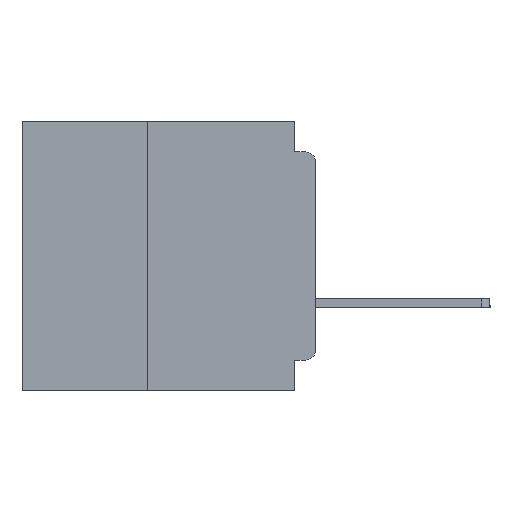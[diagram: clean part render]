
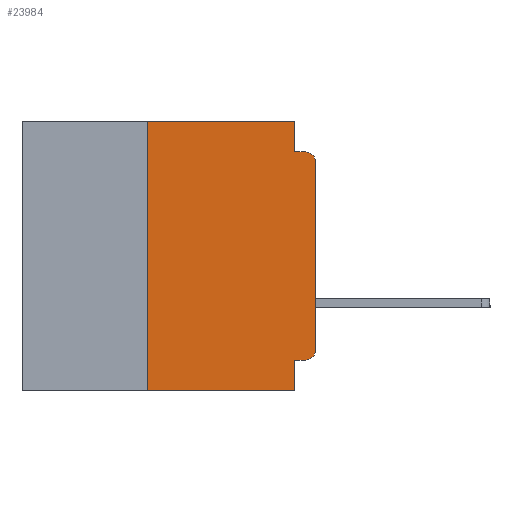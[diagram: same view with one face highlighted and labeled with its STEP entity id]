
A CAD part, left-side view. The second image highlights one B-rep face of the part: STEP entity #23984.
In plain terms, the highlighted planar face has unit normal (-1, 0, 0).
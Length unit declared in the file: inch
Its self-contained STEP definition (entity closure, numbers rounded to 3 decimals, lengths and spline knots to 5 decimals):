
#201 = ORIENTED_EDGE ( 'NONE', *, *, #36468, .T. ) ;
#619 = DIRECTION ( 'NONE',  ( 0., 1., 0. ) ) ;
#934 = CARTESIAN_POINT ( 'NONE',  ( 0., 0.25, 0. ) ) ;
#1139 = CARTESIAN_POINT ( 'NONE',  ( 0., 0.015, -0.355 ) ) ;
#1178 = CARTESIAN_POINT ( 'NONE',  ( 0., 0., -0.34 ) ) ;
#1828 = VERTEX_POINT ( 'NONE', #10863 ) ;
#1840 = CIRCLE ( 'NONE', #8574, 0.015 ) ;
#2480 = EDGE_CURVE ( 'NONE', #13129, #38058, #24101, .T. ) ;
#3026 = LINE ( 'NONE', #18519, #29274 ) ;
#3464 = LINE ( 'NONE', #41823, #29696 ) ;
#3977 = DIRECTION ( 'NONE',  ( 0., -1., 0. ) ) ;
#4245 = VERTEX_POINT ( 'NONE', #34113 ) ;
#4322 = CIRCLE ( 'NONE', #29673, 0.015 ) ;
#4446 = CARTESIAN_POINT ( 'NONE',  ( 0., 0.25, -0.4 ) ) ;
#4494 = DIRECTION ( 'NONE',  ( -1., 0., 0. ) ) ;
#4514 = CARTESIAN_POINT ( 'NONE',  ( 0., 0.437, 0. ) ) ;
#4610 = EDGE_CURVE ( 'NONE', #40332, #7298, #1840, .T. ) ;
#7077 = LINE ( 'NONE', #15061, #24202 ) ;
#7298 = VERTEX_POINT ( 'NONE', #1178 ) ;
#7424 = CARTESIAN_POINT ( 'NONE',  ( 0., 0., -0.355 ) ) ;
#8534 = ORIENTED_EDGE ( 'NONE', *, *, #34475, .F. ) ;
#8574 = AXIS2_PLACEMENT_3D ( 'NONE', #9238, #33177, #12698 ) ;
#9021 = CARTESIAN_POINT ( 'NONE',  ( 0., 0., -0.06 ) ) ;
#9238 = CARTESIAN_POINT ( 'NONE',  ( 0., 0.015, -0.34 ) ) ;
#9743 = ORIENTED_EDGE ( 'NONE', *, *, #20708, .F. ) ;
#10275 = CARTESIAN_POINT ( 'NONE',  ( 0., 0.031, 0. ) ) ;
#10671 = EDGE_CURVE ( 'NONE', #7298, #44208, #33901, .T. ) ;
#10863 = CARTESIAN_POINT ( 'NONE',  ( 0., 0.031, -0.355 ) ) ;
#11527 = EDGE_CURVE ( 'NONE', #44208, #25582, #4322, .T. ) ;
#11633 = DIRECTION ( 'NONE',  ( 0., 0., 1. ) ) ;
#12698 = DIRECTION ( 'NONE',  ( 0., 0., -1. ) ) ;
#13129 = VERTEX_POINT ( 'NONE', #934 ) ;
#13721 = CARTESIAN_POINT ( 'NONE',  ( 0., 0., 0. ) ) ;
#13884 = LINE ( 'NONE', #7424, #29902 ) ;
#15004 = VECTOR ( 'NONE', #42214, 39.37008 ) ;
#15061 = CARTESIAN_POINT ( 'NONE',  ( 0., 0.031, -0.4 ) ) ;
#16409 = VERTEX_POINT ( 'NONE', #4446 ) ;
#17164 = DIRECTION ( 'NONE',  ( 0., 0., 1. ) ) ;
#18386 = CARTESIAN_POINT ( 'NONE',  ( 0., 0.437, -0.4 ) ) ;
#18511 = DIRECTION ( 'NONE',  ( 0., 0., -1. ) ) ;
#18519 = CARTESIAN_POINT ( 'NONE',  ( 0., 0.25, -0.4 ) ) ;
#18554 = ORIENTED_EDGE ( 'NONE', *, *, #10671, .T. ) ;
#19214 = FACE_OUTER_BOUND ( 'NONE', #37015, .T. ) ;
#19450 = ORIENTED_EDGE ( 'NONE', *, *, #29506, .F. ) ;
#20221 = ORIENTED_EDGE ( 'NONE', *, *, #11527, .T. ) ;
#20708 = EDGE_CURVE ( 'NONE', #40332, #1828, #13884, .T. ) ;
#21290 = ORIENTED_EDGE ( 'NONE', *, *, #40993, .F. ) ;
#21545 = DIRECTION ( 'NONE',  ( 0., 0., -1. ) ) ;
#21841 = DIRECTION ( 'NONE',  ( 0., -1., 0. ) ) ;
#23984 = ADVANCED_FACE ( 'NONE', ( #19214 ), #35167, .F. ) ;
#24101 = LINE ( 'NONE', #4514, #15004 ) ;
#24202 = VECTOR ( 'NONE', #18511, 39.37008 ) ;
#24320 = VECTOR ( 'NONE', #41078, 39.37008 ) ;
#24983 = CARTESIAN_POINT ( 'NONE',  ( 0., 0.015, -0.06 ) ) ;
#25582 = VERTEX_POINT ( 'NONE', #37722 ) ;
#26883 = CARTESIAN_POINT ( 'NONE',  ( 0., 0.031, 0. ) ) ;
#27650 = ORIENTED_EDGE ( 'NONE', *, *, #2480, .F. ) ;
#28405 = DIRECTION ( 'NONE',  ( 0., 0., -1. ) ) ;
#29274 = VECTOR ( 'NONE', #11633, 39.37008 ) ;
#29506 = EDGE_CURVE ( 'NONE', #1828, #4245, #7077, .T. ) ;
#29673 = AXIS2_PLACEMENT_3D ( 'NONE', #24983, #4494, #28405 ) ;
#29696 = VECTOR ( 'NONE', #3977, 39.37008 ) ;
#29736 = AXIS2_PLACEMENT_3D ( 'NONE', #38573, #34885, #21545 ) ;
#29902 = VECTOR ( 'NONE', #619, 39.37008 ) ;
#31728 = VECTOR ( 'NONE', #17164, 39.37008 ) ;
#32130 = ORIENTED_EDGE ( 'NONE', *, *, #4610, .T. ) ;
#33177 = DIRECTION ( 'NONE',  ( -1., 0., 0. ) ) ;
#33901 = LINE ( 'NONE', #13721, #31728 ) ;
#34113 = CARTESIAN_POINT ( 'NONE',  ( 0., 0.031, -0.4 ) ) ;
#34475 = EDGE_CURVE ( 'NONE', #35559, #25582, #3464, .T. ) ;
#34528 = LINE ( 'NONE', #10275, #24320 ) ;
#34885 = DIRECTION ( 'NONE',  ( 1., 0., 0. ) ) ;
#35167 = PLANE ( 'NONE',  #29736 ) ;
#35559 = VERTEX_POINT ( 'NONE', #43553 ) ;
#35998 = LINE ( 'NONE', #18386, #43952 ) ;
#36468 = EDGE_CURVE ( 'NONE', #16409, #4245, #35998, .T. ) ;
#37015 = EDGE_LOOP ( 'NONE', ( #18554, #20221, #8534, #42971, #27650, #21290, #201, #19450, #9743, #32130 ) ) ;
#37722 = CARTESIAN_POINT ( 'NONE',  ( 0., 0.015, -0.045 ) ) ;
#38058 = VERTEX_POINT ( 'NONE', #26883 ) ;
#38573 = CARTESIAN_POINT ( 'NONE',  ( 0., 0.437, 0. ) ) ;
#40332 = VERTEX_POINT ( 'NONE', #1139 ) ;
#40993 = EDGE_CURVE ( 'NONE', #16409, #13129, #3026, .T. ) ;
#41078 = DIRECTION ( 'NONE',  ( 0., 0., -1. ) ) ;
#41823 = CARTESIAN_POINT ( 'NONE',  ( 0., 0., -0.045 ) ) ;
#42214 = DIRECTION ( 'NONE',  ( 0., -1., 0. ) ) ;
#42971 = ORIENTED_EDGE ( 'NONE', *, *, #43289, .F. ) ;
#43289 = EDGE_CURVE ( 'NONE', #38058, #35559, #34528, .T. ) ;
#43553 = CARTESIAN_POINT ( 'NONE',  ( 0., 0.031, -0.045 ) ) ;
#43952 = VECTOR ( 'NONE', #21841, 39.37008 ) ;
#44208 = VERTEX_POINT ( 'NONE', #9021 ) ;
